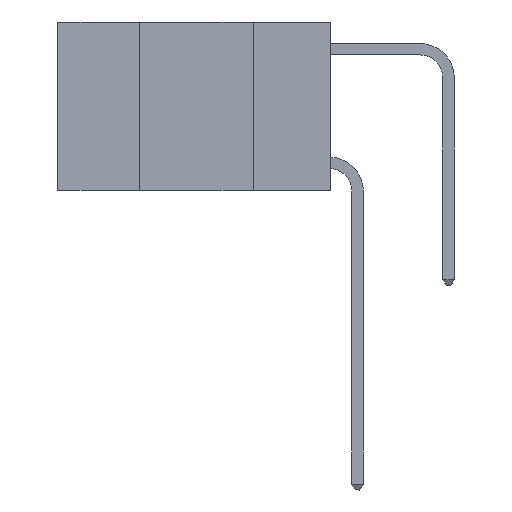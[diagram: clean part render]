
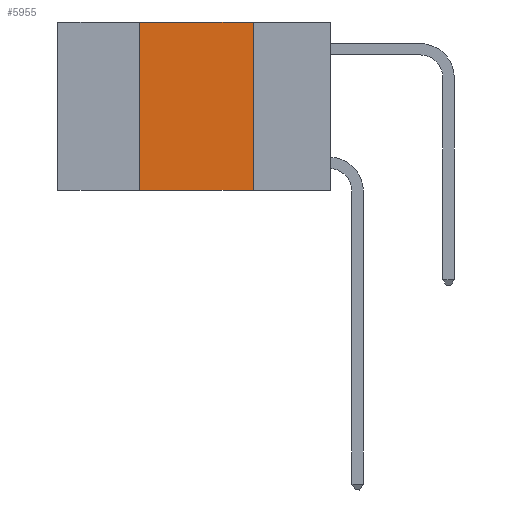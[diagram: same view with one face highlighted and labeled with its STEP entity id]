
A CAD part, left-side view. The second image highlights one B-rep face of the part: STEP entity #5955.
In plain terms, the highlighted planar face has unit normal (-1, 0, 0).
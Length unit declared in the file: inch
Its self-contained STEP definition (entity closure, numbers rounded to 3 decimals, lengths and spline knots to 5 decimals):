
#152 = ORIENTED_EDGE ( 'NONE', *, *, #167, .F. ) ;
#167 = EDGE_CURVE ( 'NONE', #10081, #4429, #1193, .T. ) ;
#985 = CARTESIAN_POINT ( 'NONE',  ( 0., 0.6, 0. ) ) ;
#1193 = LINE ( 'NONE', #6691, #12774 ) ;
#1378 = CARTESIAN_POINT ( 'NONE',  ( 0., 0.42, 0. ) ) ;
#2547 = DIRECTION ( 'NONE',  ( 0., -1., 0. ) ) ;
#2600 = DIRECTION ( 'NONE',  ( 0., 0., -1. ) ) ;
#2858 = DIRECTION ( 'NONE',  ( 0., 0., -1. ) ) ;
#4429 = VERTEX_POINT ( 'NONE', #6858 ) ;
#4841 = LINE ( 'NONE', #985, #16300 ) ;
#5955 = ADVANCED_FACE ( 'NONE', ( #12638 ), #19083, .F. ) ;
#6079 = EDGE_CURVE ( 'NONE', #14941, #13092, #10339, .T. ) ;
#6669 = ORIENTED_EDGE ( 'NONE', *, *, #6079, .F. ) ;
#6691 = CARTESIAN_POINT ( 'NONE',  ( 0., 0.17, 0. ) ) ;
#6858 = CARTESIAN_POINT ( 'NONE',  ( 0., 0.17, -0.37 ) ) ;
#9018 = VECTOR ( 'NONE', #19388, 39.37008 ) ;
#9630 = EDGE_CURVE ( 'NONE', #13092, #10081, #4841, .T. ) ;
#10081 = VERTEX_POINT ( 'NONE', #14085 ) ;
#10101 = ORIENTED_EDGE ( 'NONE', *, *, #16571, .T. ) ;
#10156 = CARTESIAN_POINT ( 'NONE',  ( 0., 0.6, 0. ) ) ;
#10339 = LINE ( 'NONE', #1378, #14723 ) ;
#11650 = DIRECTION ( 'NONE',  ( 1., 0., 0. ) ) ;
#11848 = AXIS2_PLACEMENT_3D ( 'NONE', #10156, #11650, #2600 ) ;
#11969 = DIRECTION ( 'NONE',  ( 0., 0., 1. ) ) ;
#12638 = FACE_OUTER_BOUND ( 'NONE', #13592, .T. ) ;
#12774 = VECTOR ( 'NONE', #2858, 39.37008 ) ;
#13092 = VERTEX_POINT ( 'NONE', #15993 ) ;
#13385 = LINE ( 'NONE', #14857, #9018 ) ;
#13592 = EDGE_LOOP ( 'NONE', ( #152, #18294, #6669, #10101 ) ) ;
#14016 = CARTESIAN_POINT ( 'NONE',  ( 0., 0.42, -0.37 ) ) ;
#14085 = CARTESIAN_POINT ( 'NONE',  ( 0., 0.17, 0. ) ) ;
#14723 = VECTOR ( 'NONE', #11969, 39.37008 ) ;
#14857 = CARTESIAN_POINT ( 'NONE',  ( 0., 0.6, -0.37 ) ) ;
#14941 = VERTEX_POINT ( 'NONE', #14016 ) ;
#15993 = CARTESIAN_POINT ( 'NONE',  ( 0., 0.42, 0. ) ) ;
#16300 = VECTOR ( 'NONE', #2547, 39.37008 ) ;
#16571 = EDGE_CURVE ( 'NONE', #14941, #4429, #13385, .T. ) ;
#18294 = ORIENTED_EDGE ( 'NONE', *, *, #9630, .F. ) ;
#19083 = PLANE ( 'NONE',  #11848 ) ;
#19388 = DIRECTION ( 'NONE',  ( 0., -1., 0. ) ) ;
